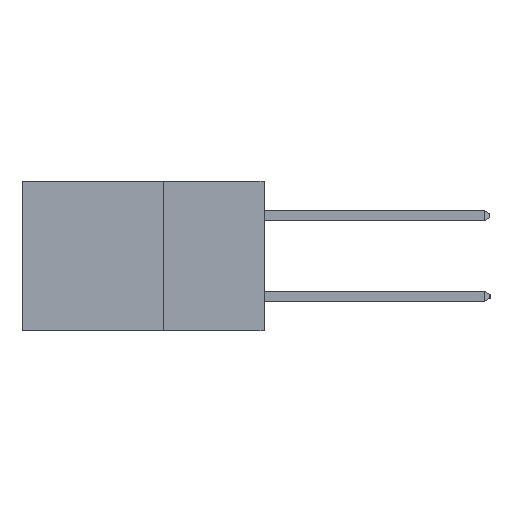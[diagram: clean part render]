
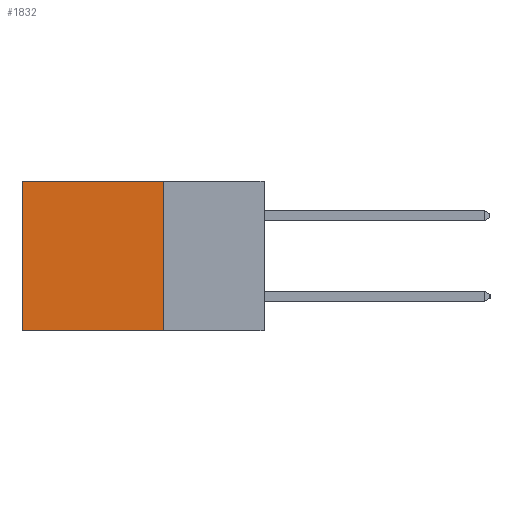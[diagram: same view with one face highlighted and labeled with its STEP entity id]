
A CAD part, left-side view. The second image highlights one B-rep face of the part: STEP entity #1832.
In plain terms, the highlighted planar face has unit normal (-1, 0, 0).
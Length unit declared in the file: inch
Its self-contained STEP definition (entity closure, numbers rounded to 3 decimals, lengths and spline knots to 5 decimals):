
#262 = CARTESIAN_POINT ( 'NONE',  ( 0.2615, 0.25, -0.37 ) ) ;
#922 = CARTESIAN_POINT ( 'NONE',  ( 0.2615, 0.6, -0.37 ) ) ;
#1503 = CARTESIAN_POINT ( 'NONE',  ( 0.2615, 0.6, 0. ) ) ;
#1620 = LINE ( 'NONE', #5206, #11709 ) ;
#1832 = ADVANCED_FACE ( 'NONE', ( #19324 ), #11106, .F. ) ;
#2945 = DIRECTION ( 'NONE',  ( 0., 1., 0. ) ) ;
#4321 = ORIENTED_EDGE ( 'NONE', *, *, #5477, .T. ) ;
#5206 = CARTESIAN_POINT ( 'NONE',  ( 0.2615, 0.25, 0. ) ) ;
#5316 = EDGE_LOOP ( 'NONE', ( #8520, #17041, #17831, #4321 ) ) ;
#5477 = EDGE_CURVE ( 'NONE', #26461, #24870, #1620, .T. ) ;
#7284 = LINE ( 'NONE', #20665, #17783 ) ;
#7652 = EDGE_CURVE ( 'NONE', #26461, #19723, #20371, .T. ) ;
#8167 = EDGE_CURVE ( 'NONE', #24870, #16966, #9239, .T. ) ;
#8520 = ORIENTED_EDGE ( 'NONE', *, *, #8167, .T. ) ;
#9239 = LINE ( 'NONE', #922, #19685 ) ;
#9656 = DIRECTION ( 'NONE',  ( 0., 0., -1. ) ) ;
#10960 = DIRECTION ( 'NONE',  ( 0., 0., -1. ) ) ;
#11023 = DIRECTION ( 'NONE',  ( 1., 0., 0. ) ) ;
#11106 = PLANE ( 'NONE',  #23903 ) ;
#11709 = VECTOR ( 'NONE', #2945, 39.37008 ) ;
#14352 = CARTESIAN_POINT ( 'NONE',  ( 0.2615, 0.25, -0.37 ) ) ;
#14408 = DIRECTION ( 'NONE',  ( 0., 0., -1. ) ) ;
#14843 = VECTOR ( 'NONE', #14408, 39.37008 ) ;
#16966 = VERTEX_POINT ( 'NONE', #24382 ) ;
#17041 = ORIENTED_EDGE ( 'NONE', *, *, #26071, .F. ) ;
#17783 = VECTOR ( 'NONE', #22757, 39.37008 ) ;
#17831 = ORIENTED_EDGE ( 'NONE', *, *, #7652, .F. ) ;
#19324 = FACE_OUTER_BOUND ( 'NONE', #5316, .T. ) ;
#19685 = VECTOR ( 'NONE', #9656, 39.37008 ) ;
#19723 = VERTEX_POINT ( 'NONE', #262 ) ;
#20371 = LINE ( 'NONE', #22691, #14843 ) ;
#20665 = CARTESIAN_POINT ( 'NONE',  ( 0.2615, 0.25, -0.37 ) ) ;
#21752 = CARTESIAN_POINT ( 'NONE',  ( 0.2615, 0.25, 0. ) ) ;
#22691 = CARTESIAN_POINT ( 'NONE',  ( 0.2615, 0.25, -0.37 ) ) ;
#22757 = DIRECTION ( 'NONE',  ( 0., 1., 0. ) ) ;
#23903 = AXIS2_PLACEMENT_3D ( 'NONE', #14352, #11023, #10960 ) ;
#24382 = CARTESIAN_POINT ( 'NONE',  ( 0.2615, 0.6, -0.37 ) ) ;
#24870 = VERTEX_POINT ( 'NONE', #1503 ) ;
#26071 = EDGE_CURVE ( 'NONE', #19723, #16966, #7284, .T. ) ;
#26461 = VERTEX_POINT ( 'NONE', #21752 ) ;
